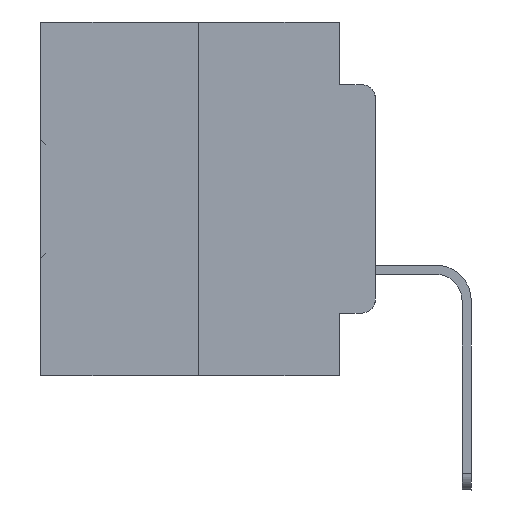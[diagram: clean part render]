
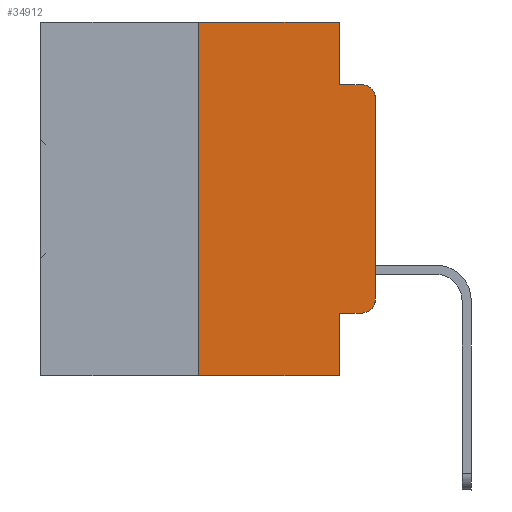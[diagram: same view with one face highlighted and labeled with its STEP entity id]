
A CAD part, left-side view. The second image highlights one B-rep face of the part: STEP entity #34912.
In plain terms, the highlighted planar face has unit normal (-1, 0, 0).
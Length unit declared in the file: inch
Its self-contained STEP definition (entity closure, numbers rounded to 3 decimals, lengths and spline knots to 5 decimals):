
#126 = AXIS2_PLACEMENT_3D ( 'NONE', #16903, #543, #25408 ) ;
#543 = DIRECTION ( 'NONE',  ( 1., 0., 0. ) ) ;
#576 = LINE ( 'NONE', #25574, #27722 ) ;
#1094 = ORIENTED_EDGE ( 'NONE', *, *, #8269, .F. ) ;
#1566 = EDGE_CURVE ( 'NONE', #32487, #17174, #33709, .T. ) ;
#1899 = DIRECTION ( 'NONE',  ( -1., 0., 0. ) ) ;
#2108 = VERTEX_POINT ( 'NONE', #22472 ) ;
#2913 = VECTOR ( 'NONE', #12672, 39.37008 ) ;
#3100 = CARTESIAN_POINT ( 'NONE',  ( 0., 0.051, -0.4115 ) ) ;
#3905 = CARTESIAN_POINT ( 'NONE',  ( 0., 0.051, -0.0885 ) ) ;
#4137 = DIRECTION ( 'NONE',  ( 0., -1., 0. ) ) ;
#5100 = VECTOR ( 'NONE', #23952, 39.37008 ) ;
#5122 = VERTEX_POINT ( 'NONE', #16985 ) ;
#5912 = EDGE_CURVE ( 'NONE', #22552, #28526, #26969, .T. ) ;
#6128 = EDGE_CURVE ( 'NONE', #34050, #6351, #24023, .T. ) ;
#6159 = ORIENTED_EDGE ( 'NONE', *, *, #5912, .F. ) ;
#6351 = VERTEX_POINT ( 'NONE', #23503 ) ;
#7000 = EDGE_CURVE ( 'NONE', #2108, #26056, #30721, .T. ) ;
#7282 = CARTESIAN_POINT ( 'NONE',  ( 0., 0.051, 0. ) ) ;
#7671 = FACE_OUTER_BOUND ( 'NONE', #17005, .T. ) ;
#8001 = VERTEX_POINT ( 'NONE', #28663 ) ;
#8205 = LINE ( 'NONE', #20702, #24296 ) ;
#8269 = EDGE_CURVE ( 'NONE', #8001, #22552, #21724, .T. ) ;
#8634 = DIRECTION ( 'NONE',  ( 0., -1., 0. ) ) ;
#8982 = PLANE ( 'NONE',  #126 ) ;
#9554 = EDGE_CURVE ( 'NONE', #8001, #17174, #576, .T. ) ;
#9663 = VECTOR ( 'NONE', #4137, 39.37008 ) ;
#11151 = VECTOR ( 'NONE', #13215, 39.37008 ) ;
#11377 = CARTESIAN_POINT ( 'NONE',  ( 0., 0., -0.3915 ) ) ;
#11965 = CARTESIAN_POINT ( 'NONE',  ( 0., 0., 0. ) ) ;
#12672 = DIRECTION ( 'NONE',  ( 0., 0., 1. ) ) ;
#13215 = DIRECTION ( 'NONE',  ( 0., 0., 1. ) ) ;
#13880 = ORIENTED_EDGE ( 'NONE', *, *, #7000, .T. ) ;
#15871 = ORIENTED_EDGE ( 'NONE', *, *, #30406, .T. ) ;
#15922 = DIRECTION ( 'NONE',  ( -1., 0., 0. ) ) ;
#15992 = CIRCLE ( 'NONE', #32348, 0.02 ) ;
#16657 = ORIENTED_EDGE ( 'NONE', *, *, #9554, .T. ) ;
#16903 = CARTESIAN_POINT ( 'NONE',  ( 0., 0.473, 0. ) ) ;
#16904 = LINE ( 'NONE', #11965, #2913 ) ;
#16985 = CARTESIAN_POINT ( 'NONE',  ( 0., 0., -0.1085 ) ) ;
#17005 = EDGE_LOOP ( 'NONE', ( #19140, #24726, #21971, #32159, #6159, #1094, #16657, #19343, #15871, #13880 ) ) ;
#17174 = VERTEX_POINT ( 'NONE', #34927 ) ;
#17186 = CARTESIAN_POINT ( 'NONE',  ( 0., 0.051, 0. ) ) ;
#17658 = DIRECTION ( 'NONE',  ( 0., 0., -1. ) ) ;
#18123 = CARTESIAN_POINT ( 'NONE',  ( 0., 0.02, -0.1085 ) ) ;
#18601 = EDGE_CURVE ( 'NONE', #26056, #5122, #16904, .T. ) ;
#19140 = ORIENTED_EDGE ( 'NONE', *, *, #18601, .T. ) ;
#19343 = ORIENTED_EDGE ( 'NONE', *, *, #1566, .F. ) ;
#19344 = AXIS2_PLACEMENT_3D ( 'NONE', #32151, #15922, #34856 ) ;
#19782 = VECTOR ( 'NONE', #8634, 39.37008 ) ;
#20490 = CARTESIAN_POINT ( 'NONE',  ( 0., 0.051, -0.0885 ) ) ;
#20702 = CARTESIAN_POINT ( 'NONE',  ( 0., 0.051, -0.4115 ) ) ;
#21724 = LINE ( 'NONE', #28965, #11151 ) ;
#21971 = ORIENTED_EDGE ( 'NONE', *, *, #6128, .F. ) ;
#22472 = CARTESIAN_POINT ( 'NONE',  ( 0., 0.02, -0.4115 ) ) ;
#22552 = VERTEX_POINT ( 'NONE', #29924 ) ;
#23493 = EDGE_CURVE ( 'NONE', #28526, #34050, #32200, .T. ) ;
#23503 = CARTESIAN_POINT ( 'NONE',  ( 0., 0.02, -0.0885 ) ) ;
#23952 = DIRECTION ( 'NONE',  ( 0., 0., -1. ) ) ;
#24023 = LINE ( 'NONE', #3905, #9663 ) ;
#24296 = VECTOR ( 'NONE', #31136, 39.37008 ) ;
#24726 = ORIENTED_EDGE ( 'NONE', *, *, #25656, .T. ) ;
#25408 = DIRECTION ( 'NONE',  ( 0., 0., -1. ) ) ;
#25574 = CARTESIAN_POINT ( 'NONE',  ( 0., 0.473, -0.5 ) ) ;
#25656 = EDGE_CURVE ( 'NONE', #5122, #6351, #15992, .T. ) ;
#26056 = VERTEX_POINT ( 'NONE', #11377 ) ;
#26969 = LINE ( 'NONE', #27341, #19782 ) ;
#27341 = CARTESIAN_POINT ( 'NONE',  ( 0., 0.473, 0. ) ) ;
#27722 = VECTOR ( 'NONE', #31031, 39.37008 ) ;
#28526 = VERTEX_POINT ( 'NONE', #31132 ) ;
#28663 = CARTESIAN_POINT ( 'NONE',  ( 0., 0.25, -0.5 ) ) ;
#28965 = CARTESIAN_POINT ( 'NONE',  ( 0., 0.25, 0. ) ) ;
#29924 = CARTESIAN_POINT ( 'NONE',  ( 0., 0.25, 0. ) ) ;
#30406 = EDGE_CURVE ( 'NONE', #32487, #2108, #8205, .T. ) ;
#30721 = CIRCLE ( 'NONE', #19344, 0.02 ) ;
#31031 = DIRECTION ( 'NONE',  ( 0., -1., 0. ) ) ;
#31132 = CARTESIAN_POINT ( 'NONE',  ( 0., 0.051, 0. ) ) ;
#31136 = DIRECTION ( 'NONE',  ( 0., -1., 0. ) ) ;
#31158 = DIRECTION ( 'NONE',  ( 0., 0., -1. ) ) ;
#32151 = CARTESIAN_POINT ( 'NONE',  ( 0., 0.02, -0.3915 ) ) ;
#32159 = ORIENTED_EDGE ( 'NONE', *, *, #23493, .F. ) ;
#32200 = LINE ( 'NONE', #7282, #5100 ) ;
#32348 = AXIS2_PLACEMENT_3D ( 'NONE', #18123, #1899, #31158 ) ;
#32487 = VERTEX_POINT ( 'NONE', #3100 ) ;
#33709 = LINE ( 'NONE', #17186, #34151 ) ;
#34050 = VERTEX_POINT ( 'NONE', #20490 ) ;
#34151 = VECTOR ( 'NONE', #17658, 39.37008 ) ;
#34856 = DIRECTION ( 'NONE',  ( 0., 0., -1. ) ) ;
#34912 = ADVANCED_FACE ( 'NONE', ( #7671 ), #8982, .F. ) ;
#34927 = CARTESIAN_POINT ( 'NONE',  ( 0., 0.051, -0.5 ) ) ;
